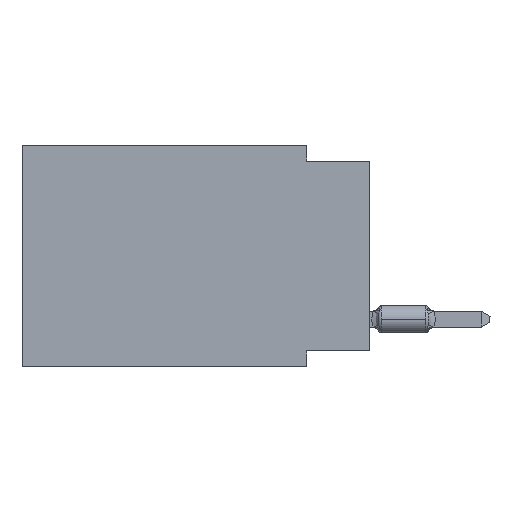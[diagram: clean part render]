
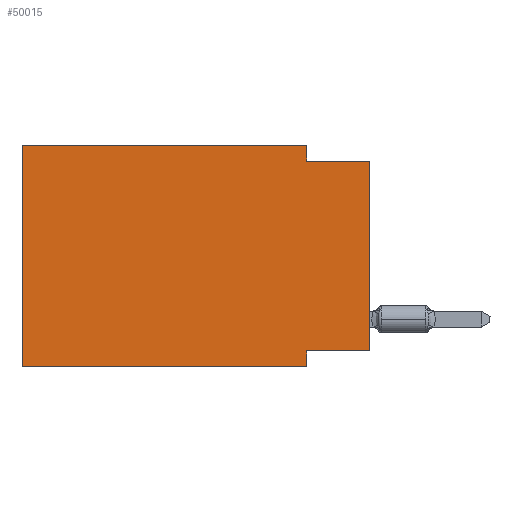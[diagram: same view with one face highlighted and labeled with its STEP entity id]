
A CAD part, left-side view. The second image highlights one B-rep face of the part: STEP entity #50015.
In plain terms, the highlighted planar face has unit normal (-1, 0, 0).
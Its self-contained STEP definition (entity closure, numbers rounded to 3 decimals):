
#5734 = ORIENTED_EDGE ( 'NONE', *, *, #84489, .F. ) ;
#6914 = DIRECTION ( 'NONE',  ( 0., 0., -1. ) ) ;
#7157 = ORIENTED_EDGE ( 'NONE', *, *, #69194, .T. ) ;
#8093 = CARTESIAN_POINT ( 'NONE',  ( 0., 0., -8.255 ) ) ;
#8151 = LINE ( 'NONE', #9055, #9121 ) ;
#8292 = EDGE_CURVE ( 'NONE', #48731, #34558, #74252, .T. ) ;
#9055 = CARTESIAN_POINT ( 'NONE',  ( 0., 13.97, 0. ) ) ;
#9121 = VECTOR ( 'NONE', #30892, 1000. ) ;
#13357 = VECTOR ( 'NONE', #48058, 1000. ) ;
#13452 = DIRECTION ( 'NONE',  ( 0., -1., 0. ) ) ;
#14408 = VERTEX_POINT ( 'NONE', #8093 ) ;
#16152 = VECTOR ( 'NONE', #46765, 1000. ) ;
#17440 = CARTESIAN_POINT ( 'NONE',  ( 0., 0., 0. ) ) ;
#20635 = EDGE_CURVE ( 'NONE', #14408, #34558, #67740, .T. ) ;
#21007 = EDGE_LOOP ( 'NONE', ( #66023, #83579, #71230, #52107, #67747, #7157, #5734, #56738 ) ) ;
#25256 = LINE ( 'NONE', #61578, #13357 ) ;
#28778 = EDGE_CURVE ( 'NONE', #29675, #48731, #44448, .T. ) ;
#28812 = VERTEX_POINT ( 'NONE', #68170 ) ;
#29675 = VERTEX_POINT ( 'NONE', #44535 ) ;
#29917 = AXIS2_PLACEMENT_3D ( 'NONE', #90282, #33037, #61454 ) ;
#30892 = DIRECTION ( 'NONE',  ( 0., 0., 1. ) ) ;
#31931 = VECTOR ( 'NONE', #39769, 1000. ) ;
#33007 = CARTESIAN_POINT ( 'NONE',  ( 0., 13.97, -8.89 ) ) ;
#33037 = DIRECTION ( 'NONE',  ( 1., 0., 0. ) ) ;
#33750 = EDGE_CURVE ( 'NONE', #14408, #82631, #25256, .T. ) ;
#34355 = CARTESIAN_POINT ( 'NONE',  ( 0., 2.54, -8.89 ) ) ;
#34558 = VERTEX_POINT ( 'NONE', #60432 ) ;
#37761 = CARTESIAN_POINT ( 'NONE',  ( 0., 2.54, -8.255 ) ) ;
#39769 = DIRECTION ( 'NONE',  ( 0., 0., -1. ) ) ;
#39988 = LINE ( 'NONE', #33007, #91579 ) ;
#40231 = CARTESIAN_POINT ( 'NONE',  ( 0., 2.54, 0. ) ) ;
#44293 = VECTOR ( 'NONE', #6914, 1000. ) ;
#44448 = LINE ( 'NONE', #40231, #31931 ) ;
#44535 = CARTESIAN_POINT ( 'NONE',  ( 0., 2.54, 0. ) ) ;
#44865 = VECTOR ( 'NONE', #45398, 1000. ) ;
#45398 = DIRECTION ( 'NONE',  ( 0., -1., 0. ) ) ;
#46765 = DIRECTION ( 'NONE',  ( 0., 0., 1. ) ) ;
#48058 = DIRECTION ( 'NONE',  ( 0., 1., 0. ) ) ;
#48731 = VERTEX_POINT ( 'NONE', #79769 ) ;
#49739 = CARTESIAN_POINT ( 'NONE',  ( 0., 13.97, 0. ) ) ;
#50015 = ADVANCED_FACE ( 'NONE', ( #81939 ), #88901, .F. ) ;
#52107 = ORIENTED_EDGE ( 'NONE', *, *, #74234, .F. ) ;
#54712 = VERTEX_POINT ( 'NONE', #91462 ) ;
#56738 = ORIENTED_EDGE ( 'NONE', *, *, #33750, .F. ) ;
#57288 = EDGE_CURVE ( 'NONE', #54712, #28812, #8151, .T. ) ;
#60432 = CARTESIAN_POINT ( 'NONE',  ( 0., 0., -0.635 ) ) ;
#61454 = DIRECTION ( 'NONE',  ( 0., 0., -1. ) ) ;
#61578 = CARTESIAN_POINT ( 'NONE',  ( 0., 0., -8.255 ) ) ;
#62642 = CARTESIAN_POINT ( 'NONE',  ( 0., 2.54, -8.89 ) ) ;
#65959 = VERTEX_POINT ( 'NONE', #62642 ) ;
#66023 = ORIENTED_EDGE ( 'NONE', *, *, #20635, .T. ) ;
#67740 = LINE ( 'NONE', #17440, #16152 ) ;
#67747 = ORIENTED_EDGE ( 'NONE', *, *, #57288, .F. ) ;
#68170 = CARTESIAN_POINT ( 'NONE',  ( 0., 13.97, 0. ) ) ;
#69194 = EDGE_CURVE ( 'NONE', #54712, #65959, #39988, .T. ) ;
#70682 = LINE ( 'NONE', #34355, #44293 ) ;
#71230 = ORIENTED_EDGE ( 'NONE', *, *, #28778, .F. ) ;
#74234 = EDGE_CURVE ( 'NONE', #28812, #29675, #79957, .T. ) ;
#74252 = LINE ( 'NONE', #88675, #44865 ) ;
#77370 = VECTOR ( 'NONE', #85569, 1000. ) ;
#79769 = CARTESIAN_POINT ( 'NONE',  ( 0., 2.54, -0.635 ) ) ;
#79957 = LINE ( 'NONE', #49739, #77370 ) ;
#81939 = FACE_OUTER_BOUND ( 'NONE', #21007, .T. ) ;
#82631 = VERTEX_POINT ( 'NONE', #37761 ) ;
#83579 = ORIENTED_EDGE ( 'NONE', *, *, #8292, .F. ) ;
#84489 = EDGE_CURVE ( 'NONE', #82631, #65959, #70682, .T. ) ;
#85569 = DIRECTION ( 'NONE',  ( 0., -1., 0. ) ) ;
#88675 = CARTESIAN_POINT ( 'NONE',  ( 0., 0., -0.635 ) ) ;
#88901 = PLANE ( 'NONE',  #29917 ) ;
#90282 = CARTESIAN_POINT ( 'NONE',  ( 0., 13.97, 0. ) ) ;
#91462 = CARTESIAN_POINT ( 'NONE',  ( 0., 13.97, -8.89 ) ) ;
#91579 = VECTOR ( 'NONE', #13452, 1000. ) ;
